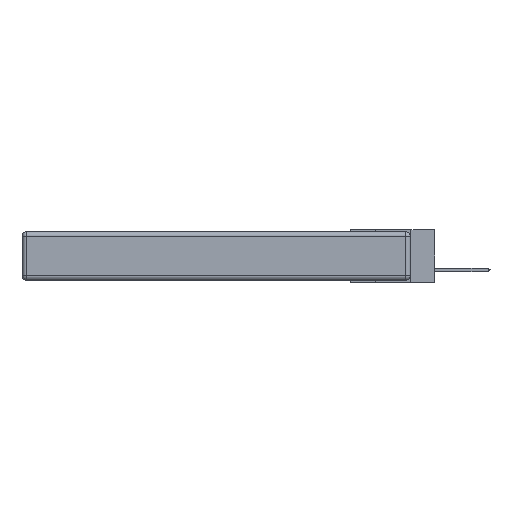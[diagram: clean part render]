
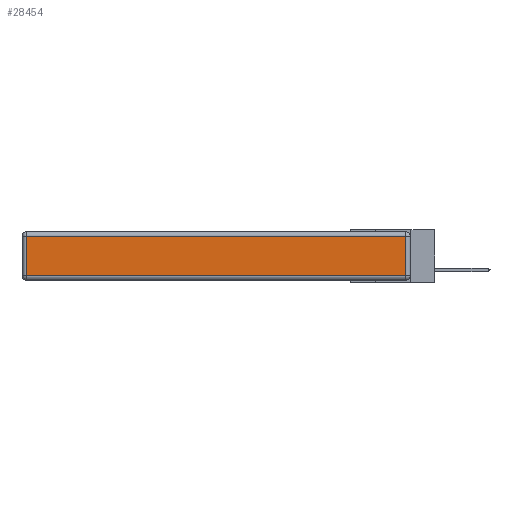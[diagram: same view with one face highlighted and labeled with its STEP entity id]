
A CAD part, left-side view. The second image highlights one B-rep face of the part: STEP entity #28454.
In plain terms, the highlighted planar face has unit normal (-1, 0, 0).
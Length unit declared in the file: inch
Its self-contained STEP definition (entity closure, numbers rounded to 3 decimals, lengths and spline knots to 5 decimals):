
#351 = EDGE_CURVE ( 'NONE', #4757, #13665, #13161, .T. ) ;
#605 = CARTESIAN_POINT ( 'NONE',  ( 0., 0.03, -0.03 ) ) ;
#1631 = ORIENTED_EDGE ( 'NONE', *, *, #351, .T. ) ;
#1936 = DIRECTION ( 'NONE',  ( 0., -1., 0. ) ) ;
#2465 = EDGE_CURVE ( 'NONE', #13665, #8883, #31191, .T. ) ;
#3767 = DIRECTION ( 'NONE',  ( 0., 0., 1. ) ) ;
#4757 = VERTEX_POINT ( 'NONE', #32173 ) ;
#4911 = EDGE_CURVE ( 'NONE', #8120, #4757, #18905, .T. ) ;
#4986 = CARTESIAN_POINT ( 'NONE',  ( 0., 2.72, -0.313 ) ) ;
#5012 = VECTOR ( 'NONE', #15257, 39.37008 ) ;
#5049 = DIRECTION ( 'NONE',  ( 0., 1., 0. ) ) ;
#5917 = VECTOR ( 'NONE', #5049, 39.37008 ) ;
#6002 = EDGE_LOOP ( 'NONE', ( #24934, #1631, #15660, #18725 ) ) ;
#6797 = CARTESIAN_POINT ( 'NONE',  ( 0., 0., -0.313 ) ) ;
#6807 = VECTOR ( 'NONE', #11946, 39.37008 ) ;
#8100 = VECTOR ( 'NONE', #1936, 39.37008 ) ;
#8120 = VERTEX_POINT ( 'NONE', #4986 ) ;
#8883 = VERTEX_POINT ( 'NONE', #27065 ) ;
#9362 = CARTESIAN_POINT ( 'NONE',  ( 0., 2.72, -0.343 ) ) ;
#11306 = PLANE ( 'NONE',  #18122 ) ;
#11651 = EDGE_CURVE ( 'NONE', #8883, #8120, #29671, .T. ) ;
#11946 = DIRECTION ( 'NONE',  ( 0., 0., -1. ) ) ;
#12008 = CARTESIAN_POINT ( 'NONE',  ( 0., 2.75, -0.03 ) ) ;
#13161 = LINE ( 'NONE', #24394, #5012 ) ;
#13665 = VERTEX_POINT ( 'NONE', #605 ) ;
#13693 = CARTESIAN_POINT ( 'NONE',  ( 0., 0., -0.343 ) ) ;
#15257 = DIRECTION ( 'NONE',  ( 0., 0., 1. ) ) ;
#15660 = ORIENTED_EDGE ( 'NONE', *, *, #2465, .T. ) ;
#18122 = AXIS2_PLACEMENT_3D ( 'NONE', #13693, #28440, #3767 ) ;
#18725 = ORIENTED_EDGE ( 'NONE', *, *, #11651, .T. ) ;
#18905 = LINE ( 'NONE', #6797, #8100 ) ;
#24394 = CARTESIAN_POINT ( 'NONE',  ( 0., 0.03, -0.343 ) ) ;
#24934 = ORIENTED_EDGE ( 'NONE', *, *, #4911, .T. ) ;
#27065 = CARTESIAN_POINT ( 'NONE',  ( 0., 2.72, -0.03 ) ) ;
#28440 = DIRECTION ( 'NONE',  ( -1., 0., 0. ) ) ;
#28454 = ADVANCED_FACE ( 'NONE', ( #30473 ), #11306, .T. ) ;
#29671 = LINE ( 'NONE', #9362, #6807 ) ;
#30473 = FACE_OUTER_BOUND ( 'NONE', #6002, .T. ) ;
#31191 = LINE ( 'NONE', #12008, #5917 ) ;
#32173 = CARTESIAN_POINT ( 'NONE',  ( 0., 0.03, -0.313 ) ) ;
